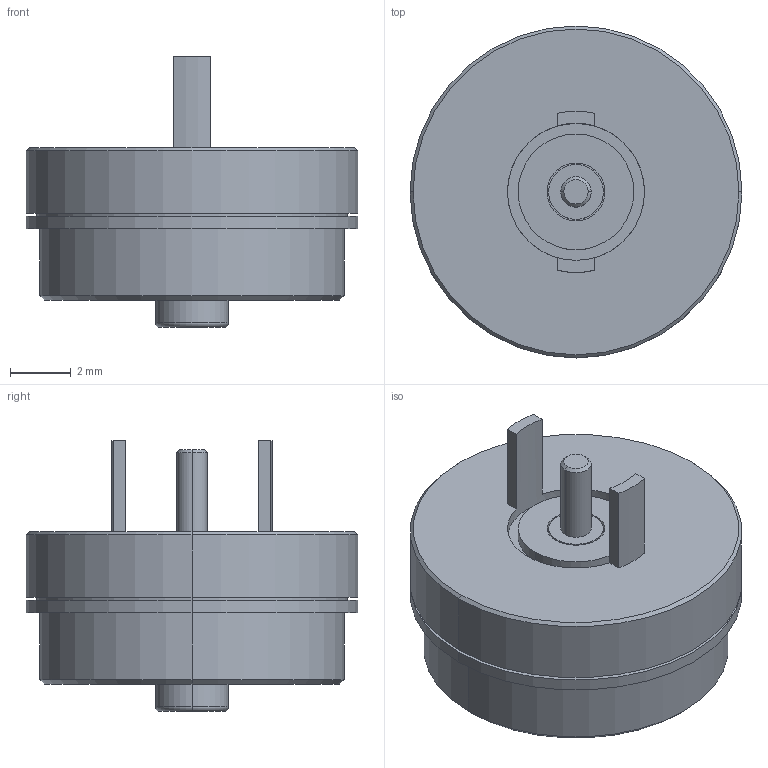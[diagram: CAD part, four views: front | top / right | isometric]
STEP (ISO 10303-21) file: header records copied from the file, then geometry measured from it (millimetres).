
FILE_DESCRIPTION (( 'STEP AP203' ), '1' );
FILE_NAME ('686-D02312030D1.STEP', '2023-02-03T17:05:02', ( 'Magnum' ), ( '' ), 'SwSTEP 2.0', 'SolidWorks 2020', '' );
FILE_SCHEMA (( 'CONFIG_CONTROL_DESIGN' ));
Length unit declared in the file: millimetre
Products named in the file (1): 686-D02312030D1
Bounding box: 10.9 x 10.9 x 8.9 mm (x, y, z)
Volume: 430 mm3; surface area: 752.8 mm2
Topology: 1 solids, 5 shells, 80 faces, 166 edges, 104 vertices
Faces by surface type: cylinder 38, plane 24, torus 10, cone 8
Entity records: 2241 total; most frequent: DIRECTION 434, CARTESIAN_POINT 351, ORIENTED_EDGE 332, AXIS2_PLACEMENT_3D 187, EDGE_CURVE 166, CIRCLE 106, VERTEX_POINT 104, EDGE_LOOP 96
